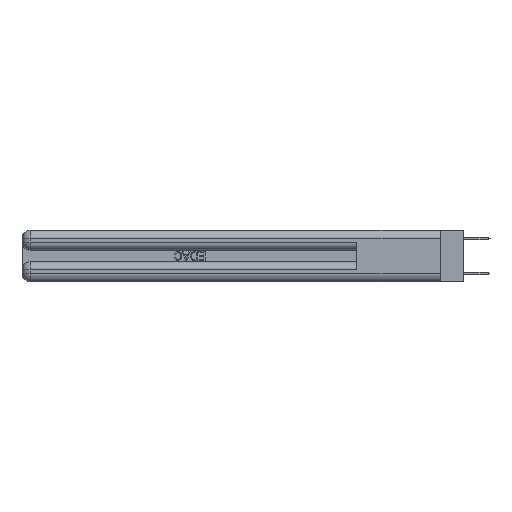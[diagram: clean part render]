
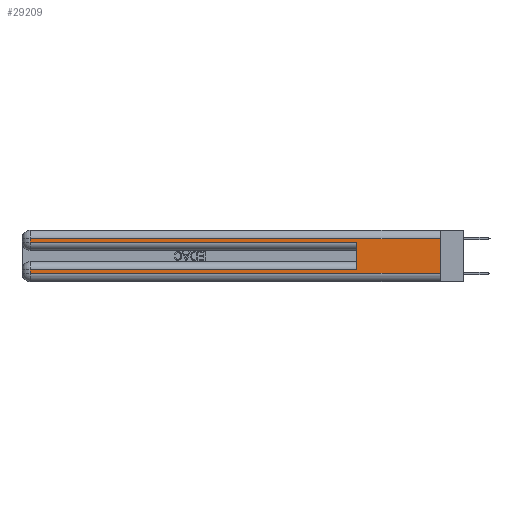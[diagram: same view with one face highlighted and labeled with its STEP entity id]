
A CAD part, left-side view. The second image highlights one B-rep face of the part: STEP entity #29209.
In plain terms, the highlighted planar face has unit normal (-1, 0, 0).
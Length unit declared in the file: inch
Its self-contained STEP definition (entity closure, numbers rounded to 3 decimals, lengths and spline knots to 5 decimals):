
#359 = LINE ( 'NONE', #13900, #18227 ) ;
#472 = CARTESIAN_POINT ( 'NONE',  ( 0., 0., 0.31 ) ) ;
#750 = ORIENTED_EDGE ( 'NONE', *, *, #18386, .T. ) ;
#811 = VERTEX_POINT ( 'NONE', #9261 ) ;
#816 = LINE ( 'NONE', #5131, #23258 ) ;
#846 = VERTEX_POINT ( 'NONE', #472 ) ;
#853 = VERTEX_POINT ( 'NONE', #29761 ) ;
#1339 = CARTESIAN_POINT ( 'NONE',  ( 0., 0., 0.31 ) ) ;
#1382 = ORIENTED_EDGE ( 'NONE', *, *, #7635, .T. ) ;
#3668 = DIRECTION ( 'NONE',  ( 0., 1., 0. ) ) ;
#4342 = CARTESIAN_POINT ( 'NONE',  ( 0., 0.6, 0.285 ) ) ;
#4474 = CARTESIAN_POINT ( 'NONE',  ( 0., 2.94, 0.37 ) ) ;
#5131 = CARTESIAN_POINT ( 'NONE',  ( 0., 0., 0.285 ) ) ;
#5171 = LINE ( 'NONE', #22423, #16850 ) ;
#6207 = VERTEX_POINT ( 'NONE', #18733 ) ;
#6343 = ORIENTED_EDGE ( 'NONE', *, *, #16123, .T. ) ;
#7635 = EDGE_CURVE ( 'NONE', #853, #29322, #18382, .T. ) ;
#7649 = CARTESIAN_POINT ( 'NONE',  ( 0., 0., 0.085 ) ) ;
#7857 = PLANE ( 'NONE',  #16467 ) ;
#7917 = VECTOR ( 'NONE', #3668, 39.37008 ) ;
#8051 = VECTOR ( 'NONE', #29638, 39.37008 ) ;
#8318 = DIRECTION ( 'NONE',  ( 0., 0., 1. ) ) ;
#9030 = ORIENTED_EDGE ( 'NONE', *, *, #25440, .T. ) ;
#9261 = CARTESIAN_POINT ( 'NONE',  ( 0., 2.94, 0.285 ) ) ;
#10266 = DIRECTION ( 'NONE',  ( 1., 0., 0. ) ) ;
#10579 = EDGE_CURVE ( 'NONE', #846, #18066, #359, .T. ) ;
#11219 = VECTOR ( 'NONE', #8318, 39.37008 ) ;
#13900 = CARTESIAN_POINT ( 'NONE',  ( 0., 0., 0.37 ) ) ;
#13985 = DIRECTION ( 'NONE',  ( 0., 0., -1. ) ) ;
#14348 = LINE ( 'NONE', #25487, #27132 ) ;
#14973 = LINE ( 'NONE', #4474, #8051 ) ;
#16123 = EDGE_CURVE ( 'NONE', #846, #21115, #26208, .T. ) ;
#16467 = AXIS2_PLACEMENT_3D ( 'NONE', #23915, #10266, #26211 ) ;
#16850 = VECTOR ( 'NONE', #24692, 39.37008 ) ;
#18066 = VERTEX_POINT ( 'NONE', #18986 ) ;
#18097 = EDGE_CURVE ( 'NONE', #811, #24942, #816, .T. ) ;
#18227 = VECTOR ( 'NONE', #27566, 39.37008 ) ;
#18382 = LINE ( 'NONE', #7649, #29642 ) ;
#18386 = EDGE_CURVE ( 'NONE', #6207, #18066, #5171, .T. ) ;
#18733 = CARTESIAN_POINT ( 'NONE',  ( 0., 2.94, 0.06 ) ) ;
#18945 = CARTESIAN_POINT ( 'NONE',  ( 0., 2.94, 0.31 ) ) ;
#18986 = CARTESIAN_POINT ( 'NONE',  ( 0., 0., 0.06 ) ) ;
#19375 = ORIENTED_EDGE ( 'NONE', *, *, #18097, .T. ) ;
#21115 = VERTEX_POINT ( 'NONE', #18945 ) ;
#21256 = ORIENTED_EDGE ( 'NONE', *, *, #23286, .T. ) ;
#21331 = EDGE_CURVE ( 'NONE', #853, #24942, #23341, .T. ) ;
#21452 = DIRECTION ( 'NONE',  ( 0., 1., 0. ) ) ;
#22423 = CARTESIAN_POINT ( 'NONE',  ( 0., 0., 0.06 ) ) ;
#23258 = VECTOR ( 'NONE', #23604, 39.37008 ) ;
#23286 = EDGE_CURVE ( 'NONE', #29322, #6207, #14348, .T. ) ;
#23341 = LINE ( 'NONE', #24255, #11219 ) ;
#23604 = DIRECTION ( 'NONE',  ( 0., -1., 0. ) ) ;
#23915 = CARTESIAN_POINT ( 'NONE',  ( 0., 0., 0.37 ) ) ;
#24124 = FACE_OUTER_BOUND ( 'NONE', #24927, .T. ) ;
#24255 = CARTESIAN_POINT ( 'NONE',  ( 0., 0.6, 0.145 ) ) ;
#24321 = CARTESIAN_POINT ( 'NONE',  ( 0., 2.94, 0.085 ) ) ;
#24692 = DIRECTION ( 'NONE',  ( 0., -1., 0. ) ) ;
#24927 = EDGE_LOOP ( 'NONE', ( #27066, #6343, #9030, #19375, #27291, #1382, #21256, #750 ) ) ;
#24942 = VERTEX_POINT ( 'NONE', #4342 ) ;
#25440 = EDGE_CURVE ( 'NONE', #21115, #811, #14973, .T. ) ;
#25487 = CARTESIAN_POINT ( 'NONE',  ( 0., 2.94, 0.37 ) ) ;
#26208 = LINE ( 'NONE', #1339, #7917 ) ;
#26211 = DIRECTION ( 'NONE',  ( 0., 0., -1. ) ) ;
#27066 = ORIENTED_EDGE ( 'NONE', *, *, #10579, .F. ) ;
#27132 = VECTOR ( 'NONE', #13985, 39.37008 ) ;
#27291 = ORIENTED_EDGE ( 'NONE', *, *, #21331, .F. ) ;
#27566 = DIRECTION ( 'NONE',  ( 0., 0., -1. ) ) ;
#29209 = ADVANCED_FACE ( 'NONE', ( #24124 ), #7857, .F. ) ;
#29322 = VERTEX_POINT ( 'NONE', #24321 ) ;
#29638 = DIRECTION ( 'NONE',  ( 0., 0., -1. ) ) ;
#29642 = VECTOR ( 'NONE', #21452, 39.37008 ) ;
#29761 = CARTESIAN_POINT ( 'NONE',  ( 0., 0.6, 0.085 ) ) ;
